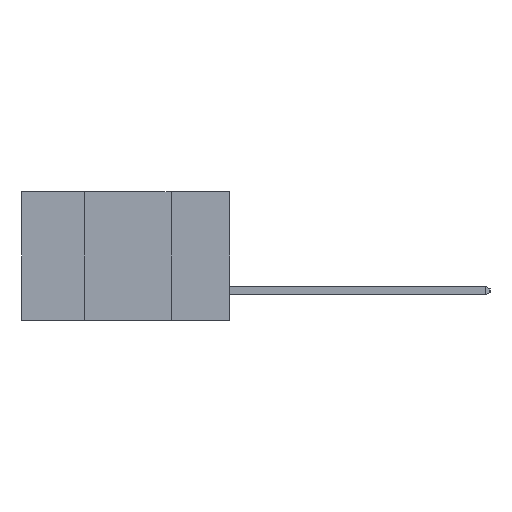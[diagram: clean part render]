
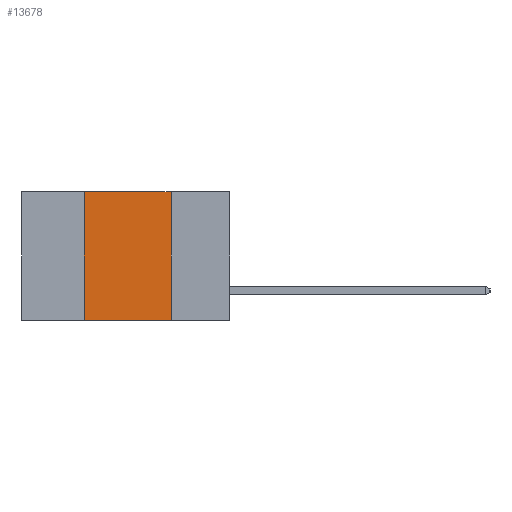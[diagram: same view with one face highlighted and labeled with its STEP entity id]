
A CAD part, left-side view. The second image highlights one B-rep face of the part: STEP entity #13678.
In plain terms, the highlighted planar face has unit normal (-1, 0, 0).
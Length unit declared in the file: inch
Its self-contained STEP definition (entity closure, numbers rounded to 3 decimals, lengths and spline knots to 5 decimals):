
#90 = CARTESIAN_POINT ( 'NONE',  ( 0., 0.42, -0.37 ) ) ;
#441 = AXIS2_PLACEMENT_3D ( 'NONE', #6556, #10979, #26644 ) ;
#4938 = CARTESIAN_POINT ( 'NONE',  ( 0., 0.17, -0.37 ) ) ;
#5233 = CARTESIAN_POINT ( 'NONE',  ( 0., 0.6, 0. ) ) ;
#5338 = DIRECTION ( 'NONE',  ( 0., 0., 1. ) ) ;
#5924 = VERTEX_POINT ( 'NONE', #13901 ) ;
#6556 = CARTESIAN_POINT ( 'NONE',  ( 0., 0.6, 0. ) ) ;
#7212 = EDGE_CURVE ( 'NONE', #5924, #14278, #13955, .T. ) ;
#7244 = EDGE_CURVE ( 'NONE', #19009, #5924, #19202, .T. ) ;
#7376 = VECTOR ( 'NONE', #7445, 39.37008 ) ;
#7445 = DIRECTION ( 'NONE',  ( 0., -1., 0. ) ) ;
#9071 = EDGE_LOOP ( 'NONE', ( #11087, #16685, #11459, #20274 ) ) ;
#10979 = DIRECTION ( 'NONE',  ( 1., 0., 0. ) ) ;
#11087 = ORIENTED_EDGE ( 'NONE', *, *, #24632, .F. ) ;
#11459 = ORIENTED_EDGE ( 'NONE', *, *, #7244, .F. ) ;
#13219 = DIRECTION ( 'NONE',  ( 0., -1., 0. ) ) ;
#13678 = ADVANCED_FACE ( 'NONE', ( #14366 ), #22140, .F. ) ;
#13792 = LINE ( 'NONE', #24497, #24336 ) ;
#13901 = CARTESIAN_POINT ( 'NONE',  ( 0., 0.42, 0. ) ) ;
#13955 = LINE ( 'NONE', #5233, #7376 ) ;
#14126 = CARTESIAN_POINT ( 'NONE',  ( 0., 0.42, 0. ) ) ;
#14261 = EDGE_CURVE ( 'NONE', #19009, #25997, #22827, .T. ) ;
#14278 = VERTEX_POINT ( 'NONE', #22226 ) ;
#14366 = FACE_OUTER_BOUND ( 'NONE', #9071, .T. ) ;
#16100 = VECTOR ( 'NONE', #13219, 39.37008 ) ;
#16685 = ORIENTED_EDGE ( 'NONE', *, *, #7212, .F. ) ;
#19009 = VERTEX_POINT ( 'NONE', #90 ) ;
#19202 = LINE ( 'NONE', #14126, #24491 ) ;
#20274 = ORIENTED_EDGE ( 'NONE', *, *, #14261, .T. ) ;
#22140 = PLANE ( 'NONE',  #441 ) ;
#22226 = CARTESIAN_POINT ( 'NONE',  ( 0., 0.17, 0. ) ) ;
#22827 = LINE ( 'NONE', #26629, #16100 ) ;
#24336 = VECTOR ( 'NONE', #26767, 39.37008 ) ;
#24491 = VECTOR ( 'NONE', #5338, 39.37008 ) ;
#24497 = CARTESIAN_POINT ( 'NONE',  ( 0., 0.17, 0. ) ) ;
#24632 = EDGE_CURVE ( 'NONE', #14278, #25997, #13792, .T. ) ;
#25997 = VERTEX_POINT ( 'NONE', #4938 ) ;
#26629 = CARTESIAN_POINT ( 'NONE',  ( 0., 0.6, -0.37 ) ) ;
#26644 = DIRECTION ( 'NONE',  ( 0., 0., -1. ) ) ;
#26767 = DIRECTION ( 'NONE',  ( 0., 0., -1. ) ) ;
